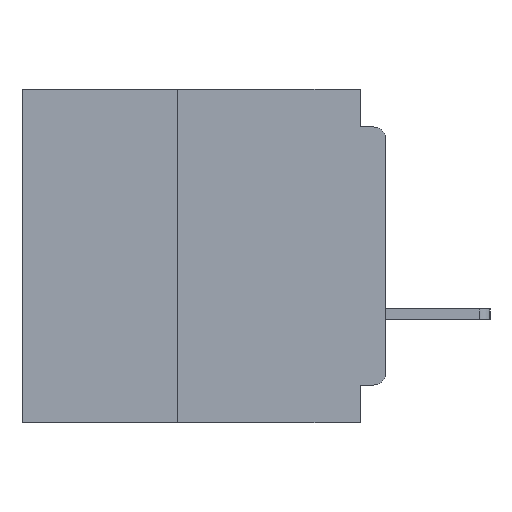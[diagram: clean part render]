
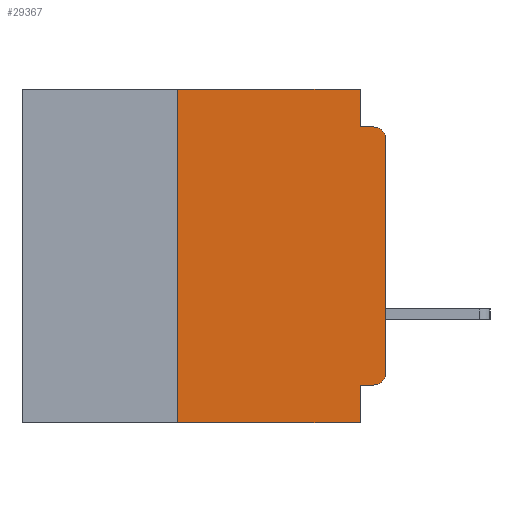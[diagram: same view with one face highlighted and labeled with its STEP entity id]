
A CAD part, left-side view. The second image highlights one B-rep face of the part: STEP entity #29367.
In plain terms, the highlighted planar face has unit normal (-1, 0, 0).
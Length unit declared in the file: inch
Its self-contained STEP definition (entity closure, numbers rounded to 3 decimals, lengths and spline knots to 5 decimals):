
#703 = DIRECTION ( 'NONE',  ( -1., 0., 0. ) ) ;
#1860 = AXIS2_PLACEMENT_3D ( 'NONE', #24511, #703, #28516 ) ;
#2246 = VECTOR ( 'NONE', #16018, 39.37008 ) ;
#2634 = VECTOR ( 'NONE', #40916, 39.37008 ) ;
#3269 = VERTEX_POINT ( 'NONE', #41708 ) ;
#4615 = ORIENTED_EDGE ( 'NONE', *, *, #37289, .F. ) ;
#4960 = ORIENTED_EDGE ( 'NONE', *, *, #43807, .T. ) ;
#8055 = LINE ( 'NONE', #44108, #39851 ) ;
#8171 = DIRECTION ( 'NONE',  ( 0., -1., 0. ) ) ;
#9299 = ORIENTED_EDGE ( 'NONE', *, *, #43498, .F. ) ;
#10497 = VERTEX_POINT ( 'NONE', #32794 ) ;
#10649 = CARTESIAN_POINT ( 'NONE',  ( 0., 0., -0.34 ) ) ;
#11538 = VECTOR ( 'NONE', #8171, 39.37008 ) ;
#11924 = ORIENTED_EDGE ( 'NONE', *, *, #43490, .F. ) ;
#12238 = CARTESIAN_POINT ( 'NONE',  ( 0., 0.031, -0.045 ) ) ;
#13139 = VECTOR ( 'NONE', #33341, 39.37008 ) ;
#14133 = EDGE_CURVE ( 'NONE', #27198, #14412, #34330, .T. ) ;
#14412 = VERTEX_POINT ( 'NONE', #15220 ) ;
#15220 = CARTESIAN_POINT ( 'NONE',  ( 0., 0.031, -0.4 ) ) ;
#15304 = LINE ( 'NONE', #31857, #2246 ) ;
#15662 = DIRECTION ( 'NONE',  ( 0., -1., 0. ) ) ;
#16018 = DIRECTION ( 'NONE',  ( 0., 0., 1. ) ) ;
#16456 = VERTEX_POINT ( 'NONE', #12238 ) ;
#16777 = VECTOR ( 'NONE', #21013, 39.37008 ) ;
#17133 = EDGE_CURVE ( 'NONE', #28710, #31732, #44003, .T. ) ;
#18516 = VECTOR ( 'NONE', #25452, 39.37008 ) ;
#19130 = LINE ( 'NONE', #39529, #39106 ) ;
#19807 = ORIENTED_EDGE ( 'NONE', *, *, #26454, .F. ) ;
#19984 = CARTESIAN_POINT ( 'NONE',  ( 0., 0., -0.045 ) ) ;
#21013 = DIRECTION ( 'NONE',  ( 0., 0., -1. ) ) ;
#21402 = FACE_OUTER_BOUND ( 'NONE', #49631, .T. ) ;
#22367 = DIRECTION ( 'NONE',  ( -1., 0., 0. ) ) ;
#22900 = PLANE ( 'NONE',  #29389 ) ;
#24511 = CARTESIAN_POINT ( 'NONE',  ( 0., 0.015, -0.34 ) ) ;
#24684 = CARTESIAN_POINT ( 'NONE',  ( 0., 0.031, 0. ) ) ;
#24885 = CARTESIAN_POINT ( 'NONE',  ( 0., 0.031, -0.355 ) ) ;
#25044 = CARTESIAN_POINT ( 'NONE',  ( 0., 0., -0.355 ) ) ;
#25452 = DIRECTION ( 'NONE',  ( 0., -1., 0. ) ) ;
#26262 = VERTEX_POINT ( 'NONE', #47658 ) ;
#26454 = EDGE_CURVE ( 'NONE', #49930, #16456, #48510, .T. ) ;
#26909 = DIRECTION ( 'NONE',  ( 0., 0., -1. ) ) ;
#27198 = VERTEX_POINT ( 'NONE', #24885 ) ;
#27711 = CARTESIAN_POINT ( 'NONE',  ( 0., 0.015, -0.045 ) ) ;
#28516 = DIRECTION ( 'NONE',  ( 0., 0., -1. ) ) ;
#28710 = VERTEX_POINT ( 'NONE', #42677 ) ;
#29367 = ADVANCED_FACE ( 'NONE', ( #21402 ), #22900, .F. ) ;
#29389 = AXIS2_PLACEMENT_3D ( 'NONE', #42781, #50730, #26909 ) ;
#29415 = ORIENTED_EDGE ( 'NONE', *, *, #45469, .F. ) ;
#30397 = ORIENTED_EDGE ( 'NONE', *, *, #17133, .T. ) ;
#31732 = VERTEX_POINT ( 'NONE', #10649 ) ;
#31857 = CARTESIAN_POINT ( 'NONE',  ( 0., 0.25, -0.4 ) ) ;
#32794 = CARTESIAN_POINT ( 'NONE',  ( 0., 0.25, 0. ) ) ;
#33341 = DIRECTION ( 'NONE',  ( 0., 0., -1. ) ) ;
#34330 = LINE ( 'NONE', #37216, #13139 ) ;
#35423 = ORIENTED_EDGE ( 'NONE', *, *, #36218, .T. ) ;
#36218 = EDGE_CURVE ( 'NONE', #31732, #3269, #8055, .T. ) ;
#37216 = CARTESIAN_POINT ( 'NONE',  ( 0., 0.031, -0.4 ) ) ;
#37289 = EDGE_CURVE ( 'NONE', #10497, #49930, #19130, .T. ) ;
#37366 = CARTESIAN_POINT ( 'NONE',  ( 0., 0.437, -0.4 ) ) ;
#37778 = AXIS2_PLACEMENT_3D ( 'NONE', #46244, #22367, #50229 ) ;
#38210 = EDGE_CURVE ( 'NONE', #26262, #14412, #40950, .T. ) ;
#38956 = CIRCLE ( 'NONE', #37778, 0.015 ) ;
#39106 = VECTOR ( 'NONE', #15662, 39.37008 ) ;
#39529 = CARTESIAN_POINT ( 'NONE',  ( 0., 0.437, 0. ) ) ;
#39851 = VECTOR ( 'NONE', #48085, 39.37008 ) ;
#40916 = DIRECTION ( 'NONE',  ( 0., 1., 0. ) ) ;
#40950 = LINE ( 'NONE', #37366, #18516 ) ;
#41708 = CARTESIAN_POINT ( 'NONE',  ( 0., 0., -0.06 ) ) ;
#42477 = LINE ( 'NONE', #25044, #2634 ) ;
#42677 = CARTESIAN_POINT ( 'NONE',  ( 0., 0.015, -0.355 ) ) ;
#42781 = CARTESIAN_POINT ( 'NONE',  ( 0., 0.437, 0. ) ) ;
#43316 = LINE ( 'NONE', #19984, #11538 ) ;
#43490 = EDGE_CURVE ( 'NONE', #26262, #10497, #15304, .T. ) ;
#43498 = EDGE_CURVE ( 'NONE', #16456, #51051, #43316, .T. ) ;
#43807 = EDGE_CURVE ( 'NONE', #3269, #51051, #38956, .T. ) ;
#44003 = CIRCLE ( 'NONE', #1860, 0.015 ) ;
#44108 = CARTESIAN_POINT ( 'NONE',  ( 0., 0., 0. ) ) ;
#44482 = ORIENTED_EDGE ( 'NONE', *, *, #38210, .T. ) ;
#44894 = CARTESIAN_POINT ( 'NONE',  ( 0., 0.031, 0. ) ) ;
#45469 = EDGE_CURVE ( 'NONE', #28710, #27198, #42477, .T. ) ;
#46244 = CARTESIAN_POINT ( 'NONE',  ( 0., 0.015, -0.06 ) ) ;
#47658 = CARTESIAN_POINT ( 'NONE',  ( 0., 0.25, -0.4 ) ) ;
#48085 = DIRECTION ( 'NONE',  ( 0., 0., 1. ) ) ;
#48510 = LINE ( 'NONE', #44894, #16777 ) ;
#49631 = EDGE_LOOP ( 'NONE', ( #35423, #4960, #9299, #19807, #4615, #11924, #44482, #50544, #29415, #30397 ) ) ;
#49930 = VERTEX_POINT ( 'NONE', #24684 ) ;
#50229 = DIRECTION ( 'NONE',  ( 0., 0., -1. ) ) ;
#50544 = ORIENTED_EDGE ( 'NONE', *, *, #14133, .F. ) ;
#50730 = DIRECTION ( 'NONE',  ( 1., 0., 0. ) ) ;
#51051 = VERTEX_POINT ( 'NONE', #27711 ) ;
